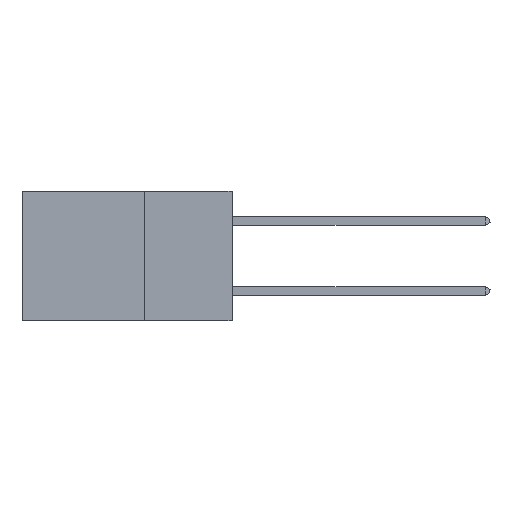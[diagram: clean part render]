
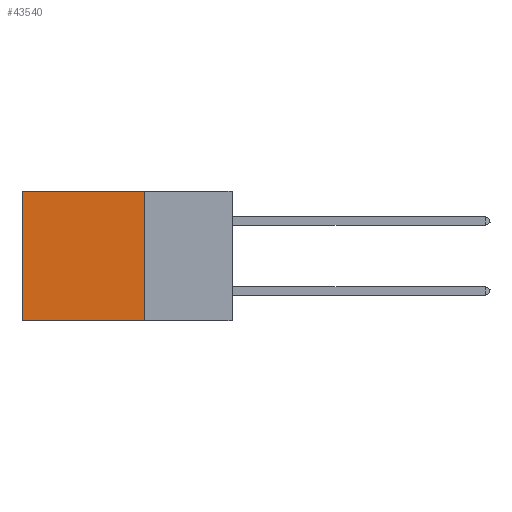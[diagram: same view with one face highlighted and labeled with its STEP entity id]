
A CAD part, left-side view. The second image highlights one B-rep face of the part: STEP entity #43540.
In plain terms, the highlighted planar face has unit normal (-1, 0, 0).
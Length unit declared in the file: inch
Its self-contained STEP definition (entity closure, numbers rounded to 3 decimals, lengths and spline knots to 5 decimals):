
#222 = LINE ( 'NONE', #41003, #17406 ) ;
#628 = VERTEX_POINT ( 'NONE', #5030 ) ;
#1957 = ORIENTED_EDGE ( 'NONE', *, *, #16743, .F. ) ;
#3282 = DIRECTION ( 'NONE',  ( 1., 0., 0. ) ) ;
#5030 = CARTESIAN_POINT ( 'NONE',  ( 0.2875, 0.6, -0.37 ) ) ;
#5176 = DIRECTION ( 'NONE',  ( 0., 1., 0. ) ) ;
#5453 = VECTOR ( 'NONE', #45626, 39.37008 ) ;
#6219 = CARTESIAN_POINT ( 'NONE',  ( 0.2875, 0.25, 0. ) ) ;
#6399 = ORIENTED_EDGE ( 'NONE', *, *, #29460, .T. ) ;
#6983 = ORIENTED_EDGE ( 'NONE', *, *, #18058, .F. ) ;
#10053 = LINE ( 'NONE', #34204, #5453 ) ;
#10309 = PLANE ( 'NONE',  #13968 ) ;
#12090 = VERTEX_POINT ( 'NONE', #25221 ) ;
#13773 = LINE ( 'NONE', #6219, #29875 ) ;
#13968 = AXIS2_PLACEMENT_3D ( 'NONE', #28663, #3282, #36059 ) ;
#14430 = FACE_OUTER_BOUND ( 'NONE', #26344, .T. ) ;
#16743 = EDGE_CURVE ( 'NONE', #12090, #19993, #222, .T. ) ;
#17406 = VECTOR ( 'NONE', #19262, 39.37008 ) ;
#18058 = EDGE_CURVE ( 'NONE', #19993, #628, #35128, .T. ) ;
#19262 = DIRECTION ( 'NONE',  ( 0., 0., -1. ) ) ;
#19993 = VERTEX_POINT ( 'NONE', #22968 ) ;
#22968 = CARTESIAN_POINT ( 'NONE',  ( 0.2875, 0.25, -0.37 ) ) ;
#25221 = CARTESIAN_POINT ( 'NONE',  ( 0.2875, 0.25, 0. ) ) ;
#25357 = DIRECTION ( 'NONE',  ( 0., 1., 0. ) ) ;
#26344 = EDGE_LOOP ( 'NONE', ( #46758, #6983, #1957, #6399 ) ) ;
#28663 = CARTESIAN_POINT ( 'NONE',  ( 0.2875, 0.25, 0. ) ) ;
#29460 = EDGE_CURVE ( 'NONE', #12090, #30796, #13773, .T. ) ;
#29875 = VECTOR ( 'NONE', #25357, 39.37008 ) ;
#30796 = VERTEX_POINT ( 'NONE', #32697 ) ;
#31779 = EDGE_CURVE ( 'NONE', #30796, #628, #10053, .T. ) ;
#32697 = CARTESIAN_POINT ( 'NONE',  ( 0.2875, 0.6, 0. ) ) ;
#34204 = CARTESIAN_POINT ( 'NONE',  ( 0.2875, 0.6, 0. ) ) ;
#35128 = LINE ( 'NONE', #45726, #38031 ) ;
#36059 = DIRECTION ( 'NONE',  ( 0., 0., -1. ) ) ;
#38031 = VECTOR ( 'NONE', #5176, 39.37008 ) ;
#41003 = CARTESIAN_POINT ( 'NONE',  ( 0.2875, 0.25, 0. ) ) ;
#43540 = ADVANCED_FACE ( 'NONE', ( #14430 ), #10309, .F. ) ;
#45626 = DIRECTION ( 'NONE',  ( 0., 0., -1. ) ) ;
#45726 = CARTESIAN_POINT ( 'NONE',  ( 0.2875, 0.25, -0.37 ) ) ;
#46758 = ORIENTED_EDGE ( 'NONE', *, *, #31779, .T. ) ;
